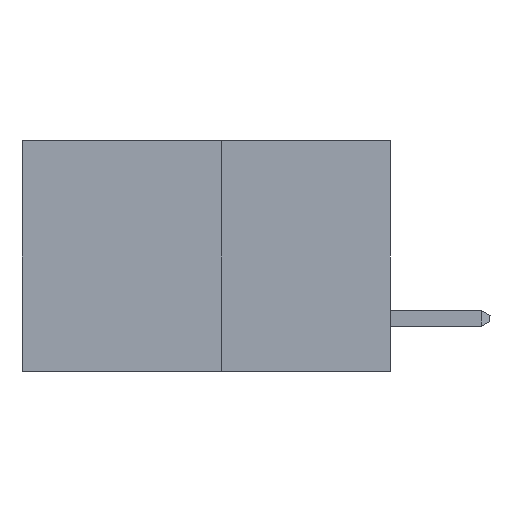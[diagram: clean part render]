
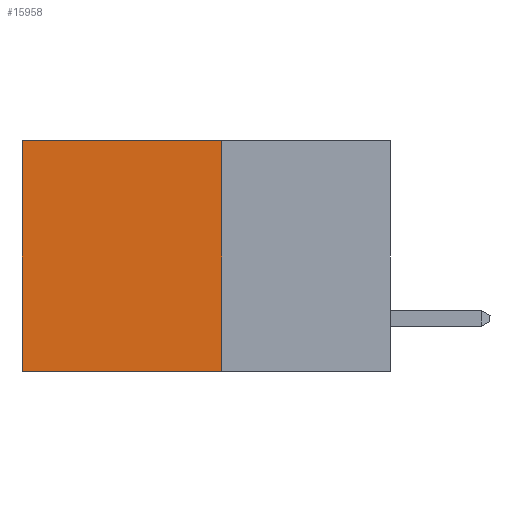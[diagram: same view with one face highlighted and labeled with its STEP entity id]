
A CAD part, left-side view. The second image highlights one B-rep face of the part: STEP entity #15958.
In plain terms, the highlighted planar face has unit normal (-1, 0, 0).
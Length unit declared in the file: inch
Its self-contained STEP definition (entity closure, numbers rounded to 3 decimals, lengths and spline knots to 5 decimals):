
#117 = PLANE ( 'NONE',  #5770 ) ;
#744 = LINE ( 'NONE', #19009, #5353 ) ;
#2152 = DIRECTION ( 'NONE',  ( 1., 0., 0. ) ) ;
#2507 = FACE_OUTER_BOUND ( 'NONE', #8849, .T. ) ;
#2721 = VECTOR ( 'NONE', #22311, 39.37008 ) ;
#2928 = VECTOR ( 'NONE', #23882, 39.37008 ) ;
#4030 = CARTESIAN_POINT ( 'NONE',  ( 0.277, 0.59, -0.37 ) ) ;
#4037 = DIRECTION ( 'NONE',  ( 0., 0., -1. ) ) ;
#4440 = VERTEX_POINT ( 'NONE', #11137 ) ;
#4485 = EDGE_CURVE ( 'NONE', #20657, #7601, #23684, .T. ) ;
#5353 = VECTOR ( 'NONE', #4037, 39.37008 ) ;
#5770 = AXIS2_PLACEMENT_3D ( 'NONE', #13509, #2152, #15452 ) ;
#6575 = ORIENTED_EDGE ( 'NONE', *, *, #20808, .T. ) ;
#7601 = VERTEX_POINT ( 'NONE', #4030 ) ;
#8174 = VERTEX_POINT ( 'NONE', #19805 ) ;
#8849 = EDGE_LOOP ( 'NONE', ( #6575, #20281, #18033, #13852 ) ) ;
#9023 = VECTOR ( 'NONE', #9265, 39.37008 ) ;
#9195 = CARTESIAN_POINT ( 'NONE',  ( 0.277, 0.27, 0. ) ) ;
#9265 = DIRECTION ( 'NONE',  ( 0., 1., 0. ) ) ;
#9999 = CARTESIAN_POINT ( 'NONE',  ( 0.277, 0.27, -0.37 ) ) ;
#11137 = CARTESIAN_POINT ( 'NONE',  ( 0.277, 0.59, 0. ) ) ;
#11365 = CARTESIAN_POINT ( 'NONE',  ( 0.277, 0.27, -0.37 ) ) ;
#12858 = LINE ( 'NONE', #20495, #2721 ) ;
#13509 = CARTESIAN_POINT ( 'NONE',  ( 0.277, 0.27, -0.37 ) ) ;
#13774 = EDGE_CURVE ( 'NONE', #8174, #4440, #23305, .T. ) ;
#13852 = ORIENTED_EDGE ( 'NONE', *, *, #13774, .T. ) ;
#15452 = DIRECTION ( 'NONE',  ( 0., 0., -1. ) ) ;
#15958 = ADVANCED_FACE ( 'NONE', ( #2507 ), #117, .F. ) ;
#18033 = ORIENTED_EDGE ( 'NONE', *, *, #24116, .F. ) ;
#19009 = CARTESIAN_POINT ( 'NONE',  ( 0.277, 0.59, -0.37 ) ) ;
#19805 = CARTESIAN_POINT ( 'NONE',  ( 0.277, 0.27, 0. ) ) ;
#20281 = ORIENTED_EDGE ( 'NONE', *, *, #4485, .F. ) ;
#20495 = CARTESIAN_POINT ( 'NONE',  ( 0.277, 0.27, -0.37 ) ) ;
#20657 = VERTEX_POINT ( 'NONE', #11365 ) ;
#20808 = EDGE_CURVE ( 'NONE', #4440, #7601, #744, .T. ) ;
#22311 = DIRECTION ( 'NONE',  ( 0., 0., -1. ) ) ;
#23305 = LINE ( 'NONE', #9195, #2928 ) ;
#23684 = LINE ( 'NONE', #9999, #9023 ) ;
#23882 = DIRECTION ( 'NONE',  ( 0., 1., 0. ) ) ;
#24116 = EDGE_CURVE ( 'NONE', #8174, #20657, #12858, .T. ) ;
